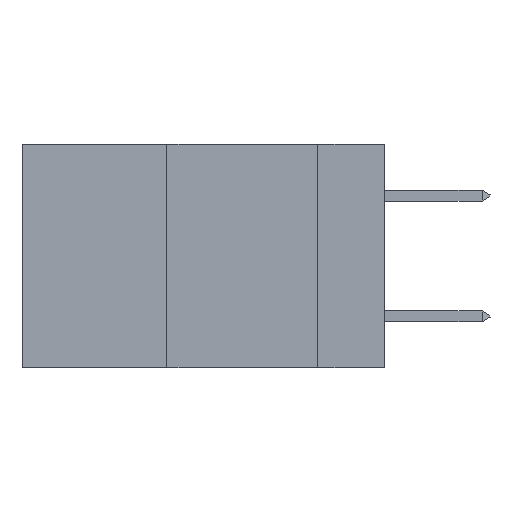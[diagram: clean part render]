
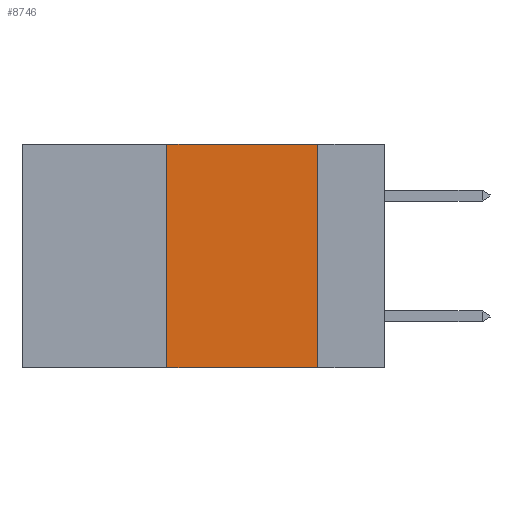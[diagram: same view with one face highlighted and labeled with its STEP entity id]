
A CAD part, left-side view. The second image highlights one B-rep face of the part: STEP entity #8746.
In plain terms, the highlighted planar face has unit normal (-1, 0, 0).
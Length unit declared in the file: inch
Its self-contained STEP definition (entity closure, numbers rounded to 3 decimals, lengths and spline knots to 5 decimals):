
#160 = VERTEX_POINT ( 'NONE', #28759 ) ;
#202 = VECTOR ( 'NONE', #2667, 39.37008 ) ;
#760 = PLANE ( 'NONE',  #9835 ) ;
#1221 = CARTESIAN_POINT ( 'NONE',  ( 0., 0.6, 0. ) ) ;
#1476 = VERTEX_POINT ( 'NONE', #7443 ) ;
#1920 = LINE ( 'NONE', #21008, #202 ) ;
#2667 = DIRECTION ( 'NONE',  ( 0., -1., 0. ) ) ;
#2772 = ORIENTED_EDGE ( 'NONE', *, *, #21288, .F. ) ;
#4030 = EDGE_CURVE ( 'NONE', #7675, #160, #8254, .T. ) ;
#5403 = DIRECTION ( 'NONE',  ( 0., 0., -1. ) ) ;
#6725 = VERTEX_POINT ( 'NONE', #9484 ) ;
#7377 = VECTOR ( 'NONE', #32665, 39.37008 ) ;
#7443 = CARTESIAN_POINT ( 'NONE',  ( 0., 0.11, 0. ) ) ;
#7675 = VERTEX_POINT ( 'NONE', #25390 ) ;
#8254 = LINE ( 'NONE', #24543, #30772 ) ;
#8746 = ADVANCED_FACE ( 'NONE', ( #14089 ), #760, .F. ) ;
#8832 = DIRECTION ( 'NONE',  ( 1., 0., 0. ) ) ;
#8974 = ORIENTED_EDGE ( 'NONE', *, *, #4030, .F. ) ;
#9484 = CARTESIAN_POINT ( 'NONE',  ( 0., 0.11, -0.37 ) ) ;
#9558 = ORIENTED_EDGE ( 'NONE', *, *, #21664, .T. ) ;
#9835 = AXIS2_PLACEMENT_3D ( 'NONE', #1221, #8832, #25018 ) ;
#14089 = FACE_OUTER_BOUND ( 'NONE', #14515, .T. ) ;
#14515 = EDGE_LOOP ( 'NONE', ( #23864, #2772, #8974, #9558 ) ) ;
#16525 = LINE ( 'NONE', #19610, #7377 ) ;
#18942 = LINE ( 'NONE', #29448, #19357 ) ;
#19357 = VECTOR ( 'NONE', #5403, 39.37008 ) ;
#19610 = CARTESIAN_POINT ( 'NONE',  ( 0., 0.6, 0. ) ) ;
#21008 = CARTESIAN_POINT ( 'NONE',  ( 0., 0.6, -0.37 ) ) ;
#21288 = EDGE_CURVE ( 'NONE', #160, #1476, #16525, .T. ) ;
#21664 = EDGE_CURVE ( 'NONE', #7675, #6725, #1920, .T. ) ;
#22911 = EDGE_CURVE ( 'NONE', #1476, #6725, #18942, .T. ) ;
#23864 = ORIENTED_EDGE ( 'NONE', *, *, #22911, .F. ) ;
#24543 = CARTESIAN_POINT ( 'NONE',  ( 0., 0.36, 0. ) ) ;
#25018 = DIRECTION ( 'NONE',  ( 0., 0., -1. ) ) ;
#25390 = CARTESIAN_POINT ( 'NONE',  ( 0., 0.36, -0.37 ) ) ;
#28759 = CARTESIAN_POINT ( 'NONE',  ( 0., 0.36, 0. ) ) ;
#29448 = CARTESIAN_POINT ( 'NONE',  ( 0., 0.11, 0. ) ) ;
#30281 = DIRECTION ( 'NONE',  ( 0., 0., 1. ) ) ;
#30772 = VECTOR ( 'NONE', #30281, 39.37008 ) ;
#32665 = DIRECTION ( 'NONE',  ( 0., -1., 0. ) ) ;
